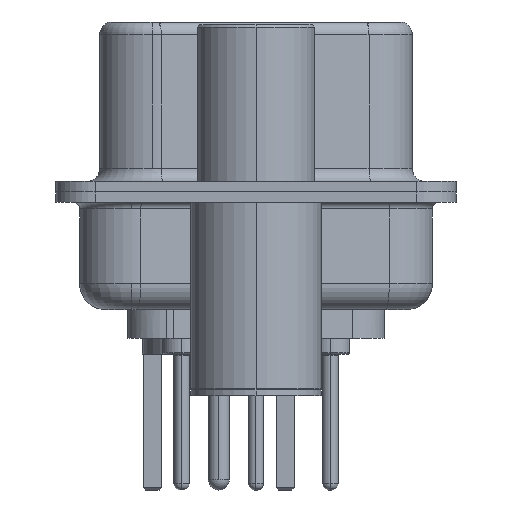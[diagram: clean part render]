
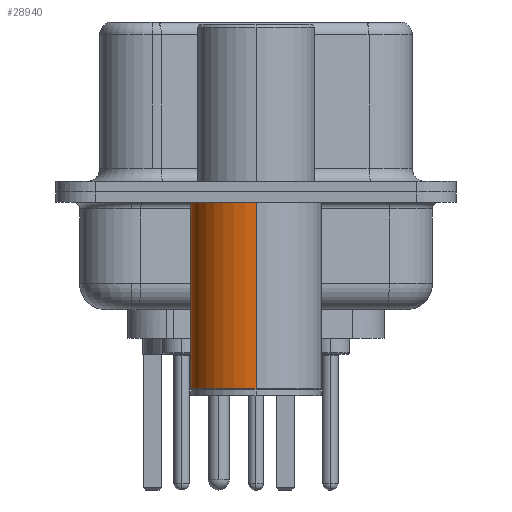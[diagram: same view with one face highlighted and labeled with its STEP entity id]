
A CAD part, left-side view. The second image highlights one B-rep face of the part: STEP entity #28940.
In plain terms, the highlighted cylindrical face has radius 2.5 mm (diameter 5 mm), a partial arc.
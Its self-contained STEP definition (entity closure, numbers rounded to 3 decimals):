
#691 = FACE_OUTER_BOUND ( 'NONE', #20698, .T. ) ;
#885 = ORIENTED_EDGE ( 'NONE', *, *, #30266, .T. ) ;
#2491 = CARTESIAN_POINT ( 'NONE',  ( 2.5, 0., -0.4 ) ) ;
#2601 = VECTOR ( 'NONE', #28983, 1000. ) ;
#2743 = DIRECTION ( 'NONE',  ( 1., 0., 0. ) ) ;
#5491 = DIRECTION ( 'NONE',  ( 0., 0., 1. ) ) ;
#7407 = DIRECTION ( 'NONE',  ( 0., 0., 1. ) ) ;
#7853 = ORIENTED_EDGE ( 'NONE', *, *, #9251, .F. ) ;
#9251 = EDGE_CURVE ( 'NONE', #25495, #14217, #15197, .T. ) ;
#13986 = AXIS2_PLACEMENT_3D ( 'NONE', #18827, #5491, #2743 ) ;
#14217 = VERTEX_POINT ( 'NONE', #2491 ) ;
#14337 = DIRECTION ( 'NONE',  ( 1., 0., 0. ) ) ;
#15197 = LINE ( 'NONE', #25232, #17711 ) ;
#15605 = ORIENTED_EDGE ( 'NONE', *, *, #28317, .F. ) ;
#15878 = CARTESIAN_POINT ( 'NONE',  ( 0., 0., -0.4 ) ) ;
#15984 = DIRECTION ( 'NONE',  ( 0., 0., 1. ) ) ;
#16426 = CIRCLE ( 'NONE', #13986, 2.5 ) ;
#17711 = VECTOR ( 'NONE', #33331, 1000. ) ;
#18546 = DIRECTION ( 'NONE',  ( 1., 0., 0. ) ) ;
#18827 = CARTESIAN_POINT ( 'NONE',  ( 0., 0., -7.525 ) ) ;
#19247 = CARTESIAN_POINT ( 'NONE',  ( 2.5, 0., -7.525 ) ) ;
#20698 = EDGE_LOOP ( 'NONE', ( #29802, #885, #15605, #7853 ) ) ;
#21833 = EDGE_CURVE ( 'NONE', #25495, #24696, #16426, .T. ) ;
#22122 = CIRCLE ( 'NONE', #28738, 2.5 ) ;
#23689 = CARTESIAN_POINT ( 'NONE',  ( -2.5, 0., 0.581 ) ) ;
#24696 = VERTEX_POINT ( 'NONE', #29425 ) ;
#25232 = CARTESIAN_POINT ( 'NONE',  ( 2.5, 0., 0.581 ) ) ;
#25495 = VERTEX_POINT ( 'NONE', #19247 ) ;
#26872 = LINE ( 'NONE', #23689, #2601 ) ;
#27195 = CARTESIAN_POINT ( 'NONE',  ( -2.5, 0., -0.4 ) ) ;
#28317 = EDGE_CURVE ( 'NONE', #14217, #28595, #22122, .T. ) ;
#28595 = VERTEX_POINT ( 'NONE', #27195 ) ;
#28738 = AXIS2_PLACEMENT_3D ( 'NONE', #15878, #15984, #18546 ) ;
#28828 = AXIS2_PLACEMENT_3D ( 'NONE', #32528, #7407, #14337 ) ;
#28940 = ADVANCED_FACE ( 'NONE', ( #691 ), #30651, .T. ) ;
#28983 = DIRECTION ( 'NONE',  ( 0., 0., 1. ) ) ;
#29425 = CARTESIAN_POINT ( 'NONE',  ( -2.5, 0., -7.525 ) ) ;
#29802 = ORIENTED_EDGE ( 'NONE', *, *, #21833, .T. ) ;
#30266 = EDGE_CURVE ( 'NONE', #24696, #28595, #26872, .T. ) ;
#30651 = CYLINDRICAL_SURFACE ( 'NONE', #28828, 2.5 ) ;
#32528 = CARTESIAN_POINT ( 'NONE',  ( 0., 0., 0.581 ) ) ;
#33331 = DIRECTION ( 'NONE',  ( 0., 0., 1. ) ) ;
